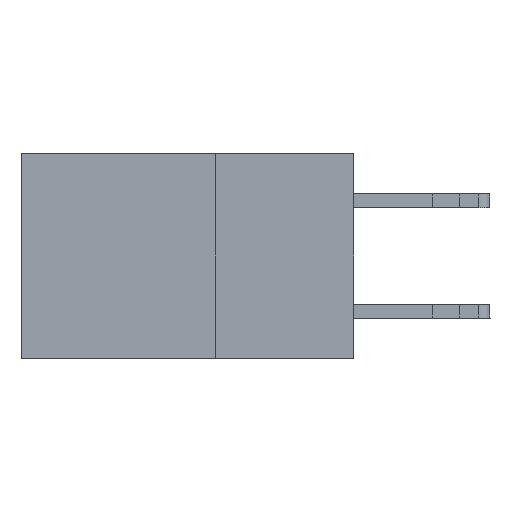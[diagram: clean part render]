
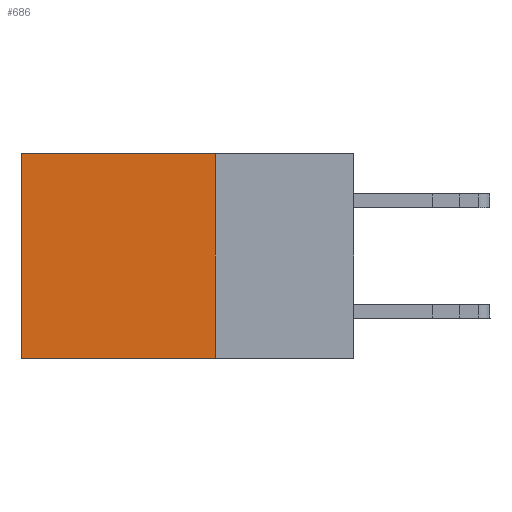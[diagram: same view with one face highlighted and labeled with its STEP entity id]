
A CAD part, left-side view. The second image highlights one B-rep face of the part: STEP entity #686.
In plain terms, the highlighted planar face has unit normal (-1, 0, 0).
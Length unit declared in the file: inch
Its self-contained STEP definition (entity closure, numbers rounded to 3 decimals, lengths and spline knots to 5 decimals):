
#686 = ADVANCED_FACE ( 'NONE', ( #10667 ), #4004, .F. ) ;
#801 = EDGE_CURVE ( 'NONE', #4937, #14698, #14560, .T. ) ;
#1318 = CARTESIAN_POINT ( 'NONE',  ( 0.2875, 0.25, -0.37 ) ) ;
#1646 = EDGE_CURVE ( 'NONE', #4937, #3828, #4209, .T. ) ;
#2041 = VECTOR ( 'NONE', #9439, 39.37008 ) ;
#2393 = DIRECTION ( 'NONE',  ( 0., 0., -1. ) ) ;
#2497 = VECTOR ( 'NONE', #12334, 39.37008 ) ;
#2525 = DIRECTION ( 'NONE',  ( 0., 0., -1. ) ) ;
#3685 = EDGE_LOOP ( 'NONE', ( #21683, #20356, #14848, #20876 ) ) ;
#3828 = VERTEX_POINT ( 'NONE', #20095 ) ;
#4004 = PLANE ( 'NONE',  #18691 ) ;
#4209 = LINE ( 'NONE', #20671, #2497 ) ;
#4577 = VECTOR ( 'NONE', #2393, 39.37008 ) ;
#4625 = DIRECTION ( 'NONE',  ( 0., 0., -1. ) ) ;
#4937 = VERTEX_POINT ( 'NONE', #16195 ) ;
#6136 = CARTESIAN_POINT ( 'NONE',  ( 0.2875, 0.25, -0.37 ) ) ;
#9439 = DIRECTION ( 'NONE',  ( 0., 1., 0. ) ) ;
#10391 = EDGE_CURVE ( 'NONE', #3828, #26025, #17330, .T. ) ;
#10667 = FACE_OUTER_BOUND ( 'NONE', #3685, .T. ) ;
#12334 = DIRECTION ( 'NONE',  ( 0., 1., 0. ) ) ;
#13285 = CARTESIAN_POINT ( 'NONE',  ( 0.2875, 0.6, 0. ) ) ;
#14560 = LINE ( 'NONE', #22679, #4577 ) ;
#14698 = VERTEX_POINT ( 'NONE', #6136 ) ;
#14848 = ORIENTED_EDGE ( 'NONE', *, *, #801, .F. ) ;
#16195 = CARTESIAN_POINT ( 'NONE',  ( 0.2875, 0.25, 0. ) ) ;
#16330 = CARTESIAN_POINT ( 'NONE',  ( 0.2875, 0.25, 0. ) ) ;
#17330 = LINE ( 'NONE', #13285, #24915 ) ;
#18691 = AXIS2_PLACEMENT_3D ( 'NONE', #16330, #24938, #2525 ) ;
#19517 = EDGE_CURVE ( 'NONE', #14698, #26025, #19630, .T. ) ;
#19630 = LINE ( 'NONE', #1318, #2041 ) ;
#20095 = CARTESIAN_POINT ( 'NONE',  ( 0.2875, 0.6, 0. ) ) ;
#20356 = ORIENTED_EDGE ( 'NONE', *, *, #19517, .F. ) ;
#20671 = CARTESIAN_POINT ( 'NONE',  ( 0.2875, 0.25, 0. ) ) ;
#20876 = ORIENTED_EDGE ( 'NONE', *, *, #1646, .T. ) ;
#21683 = ORIENTED_EDGE ( 'NONE', *, *, #10391, .T. ) ;
#22679 = CARTESIAN_POINT ( 'NONE',  ( 0.2875, 0.25, 0. ) ) ;
#24915 = VECTOR ( 'NONE', #4625, 39.37008 ) ;
#24938 = DIRECTION ( 'NONE',  ( 1., 0., 0. ) ) ;
#25131 = CARTESIAN_POINT ( 'NONE',  ( 0.2875, 0.6, -0.37 ) ) ;
#26025 = VERTEX_POINT ( 'NONE', #25131 ) ;
